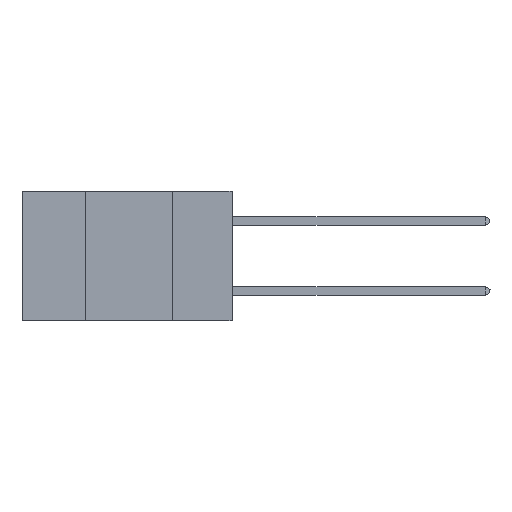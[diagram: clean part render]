
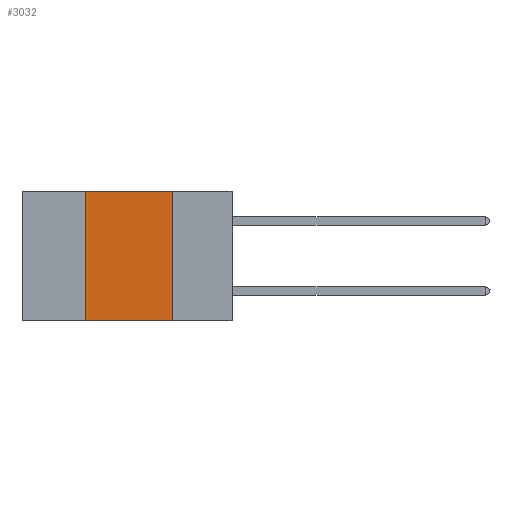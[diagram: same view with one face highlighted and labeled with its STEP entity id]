
A CAD part, left-side view. The second image highlights one B-rep face of the part: STEP entity #3032.
In plain terms, the highlighted planar face has unit normal (-1, 0, 0).
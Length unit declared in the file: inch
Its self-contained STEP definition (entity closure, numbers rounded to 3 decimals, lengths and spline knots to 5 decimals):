
#1929 = VERTEX_POINT ( 'NONE', #13135 ) ;
#3032 = ADVANCED_FACE ( 'NONE', ( #37100 ), #8119, .F. ) ;
#3222 = CARTESIAN_POINT ( 'NONE',  ( 0., 0.6, -0.37 ) ) ;
#4111 = EDGE_CURVE ( 'NONE', #31273, #20139, #35528, .T. ) ;
#4547 = EDGE_CURVE ( 'NONE', #1929, #20139, #10506, .T. ) ;
#6980 = EDGE_CURVE ( 'NONE', #18876, #1929, #25594, .T. ) ;
#7101 = EDGE_LOOP ( 'NONE', ( #26294, #26919, #13226, #9493 ) ) ;
#7851 = CARTESIAN_POINT ( 'NONE',  ( 0., 0.17, -0.37 ) ) ;
#8119 = PLANE ( 'NONE',  #39666 ) ;
#8203 = CARTESIAN_POINT ( 'NONE',  ( 0., 0.17, 0. ) ) ;
#8209 = DIRECTION ( 'NONE',  ( 0., -1., 0. ) ) ;
#8489 = DIRECTION ( 'NONE',  ( 0., 0., -1. ) ) ;
#9377 = DIRECTION ( 'NONE',  ( 0., 0., 1. ) ) ;
#9493 = ORIENTED_EDGE ( 'NONE', *, *, #4111, .T. ) ;
#10506 = LINE ( 'NONE', #8203, #30915 ) ;
#11554 = DIRECTION ( 'NONE',  ( 0., 0., -1. ) ) ;
#12216 = VECTOR ( 'NONE', #9377, 39.37008 ) ;
#13135 = CARTESIAN_POINT ( 'NONE',  ( 0., 0.17, 0. ) ) ;
#13226 = ORIENTED_EDGE ( 'NONE', *, *, #41024, .F. ) ;
#13237 = LINE ( 'NONE', #35596, #12216 ) ;
#13653 = VECTOR ( 'NONE', #30012, 39.37008 ) ;
#18876 = VERTEX_POINT ( 'NONE', #24862 ) ;
#20139 = VERTEX_POINT ( 'NONE', #7851 ) ;
#24862 = CARTESIAN_POINT ( 'NONE',  ( 0., 0.42, 0. ) ) ;
#25594 = LINE ( 'NONE', #40420, #34753 ) ;
#26294 = ORIENTED_EDGE ( 'NONE', *, *, #4547, .F. ) ;
#26919 = ORIENTED_EDGE ( 'NONE', *, *, #6980, .F. ) ;
#27919 = CARTESIAN_POINT ( 'NONE',  ( 0., 0.6, 0. ) ) ;
#30012 = DIRECTION ( 'NONE',  ( 0., -1., 0. ) ) ;
#30915 = VECTOR ( 'NONE', #8489, 39.37008 ) ;
#31273 = VERTEX_POINT ( 'NONE', #31950 ) ;
#31950 = CARTESIAN_POINT ( 'NONE',  ( 0., 0.42, -0.37 ) ) ;
#34181 = DIRECTION ( 'NONE',  ( 1., 0., 0. ) ) ;
#34753 = VECTOR ( 'NONE', #8209, 39.37008 ) ;
#35528 = LINE ( 'NONE', #3222, #13653 ) ;
#35596 = CARTESIAN_POINT ( 'NONE',  ( 0., 0.42, 0. ) ) ;
#37100 = FACE_OUTER_BOUND ( 'NONE', #7101, .T. ) ;
#39666 = AXIS2_PLACEMENT_3D ( 'NONE', #27919, #34181, #11554 ) ;
#40420 = CARTESIAN_POINT ( 'NONE',  ( 0., 0.6, 0. ) ) ;
#41024 = EDGE_CURVE ( 'NONE', #31273, #18876, #13237, .T. ) ;
